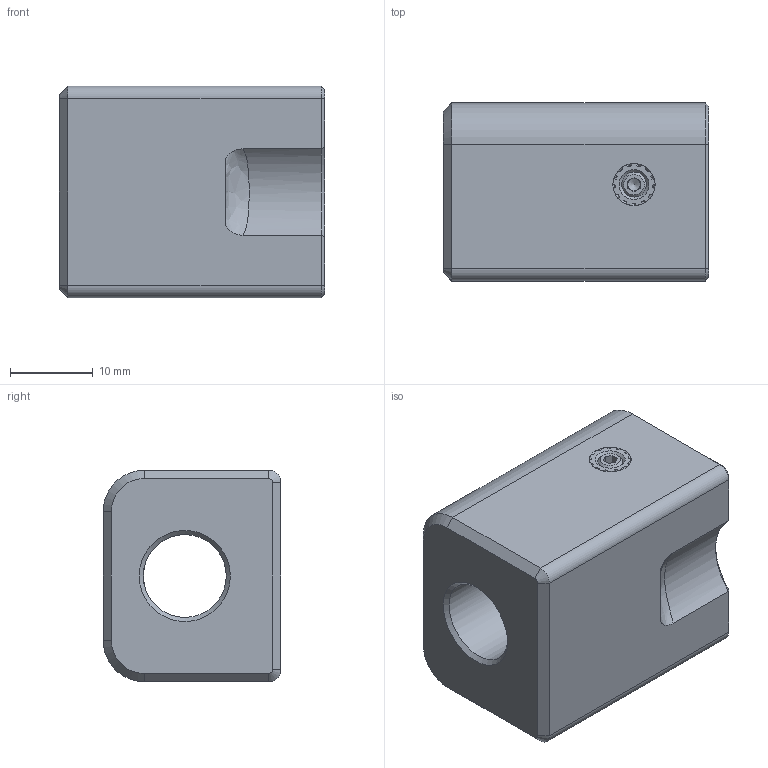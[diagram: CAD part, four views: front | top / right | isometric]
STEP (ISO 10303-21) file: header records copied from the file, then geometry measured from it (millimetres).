
FILE_DESCRIPTION(/* description */ (''),/* implementation_level */ '2;1');
FILE_NAME(/* name */ 'Glock Minor Comp.step',/* time_stamp */ '2023-01-27T20:02:09+13:00',/* author */ (''),/* organization */ (''),/* preprocessor_version */ 'ST-DEVELOPER v19.2',/* originating_system */ 'Autodesk Translation Framework v11.17.0.187',/* authorisation */ '');
FILE_SCHEMA (('AUTOMOTIVE_DESIGN { 1 0 10303 214 3 1 1 }'));
Length unit declared in the file: millimetre
Products named in the file (3): Glock Minor Comp; VORON2.4_Assembly_M3 Threaded Insert; SBCP3-6 v2
Assembly tree (4 placements, depth 2):
  Glock Minor Comp
    VORON2.4_Assembly_M3 Threaded Insert  x2
    SBCP3-6 v2  x2
Bounding box: 32 x 21.46 x 25.53 mm (x, y, z)
Volume: 13299.4 mm3; surface area: 5529.1 mm2
Topology: 5 solids, 5 shells, 377 faces, 1026 edges, 664 vertices
Faces by surface type: bspline 177, cylinder 106, plane 62, cone 29, torus 3
Full cylindrical faces by diameter (mm): 1.5 x2, 2.9 x2, 3 x2, 3.4 x2, 4.2 x2, 4.25 x2, 4.6 x2, 4.7 x2, 10 x1, 11.793 x4, 12.7 x4, 14.6 x1
Entity records: 12160 total; most frequent: CARTESIAN_POINT 6994, ORIENTED_EDGE 1294, DIRECTION 667, EDGE_CURVE 647, VERTEX_POINT 418, B_SPLINE_CURVE_WITH_KNOTS 403, AXIS2_PLACEMENT_3D 275, EDGE_LOOP 255
